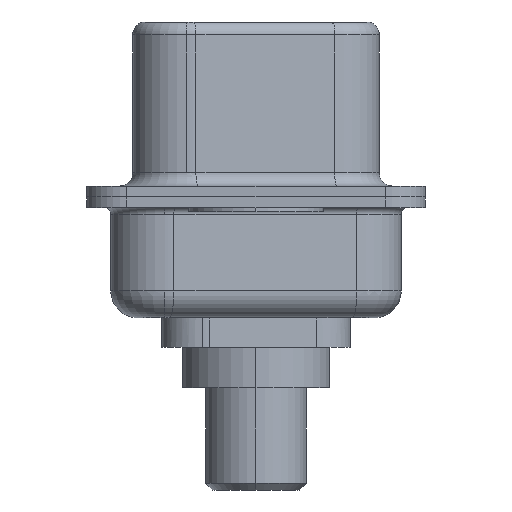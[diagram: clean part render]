
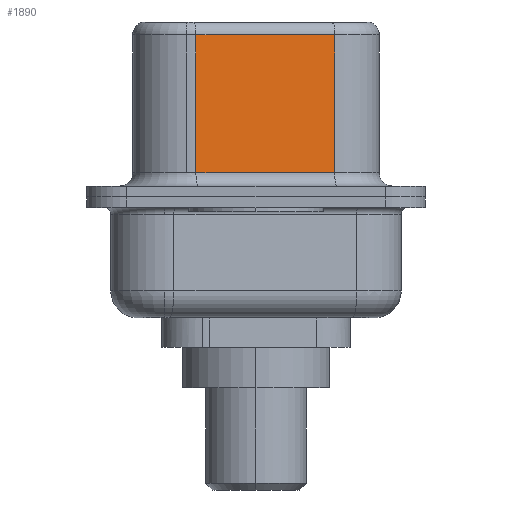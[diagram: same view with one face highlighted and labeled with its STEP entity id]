
A CAD part, left-side view. The second image highlights one B-rep face of the part: STEP entity #1890.
In plain terms, the highlighted planar face has unit normal (-0.985, -0.174, 0).
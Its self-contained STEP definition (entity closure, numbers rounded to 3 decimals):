
#310 = CARTESIAN_POINT ( 'NONE',  ( 4.585, -2.927, 6.02 ) ) ;
#383 = DIRECTION ( 'NONE',  ( -0.174, 0.985, 0. ) ) ;
#447 = DIRECTION ( 'NONE',  ( 0., 0., -1. ) ) ;
#1462 = EDGE_CURVE ( 'NONE', #12313, #4201, #1863, .T. ) ;
#1636 = ORIENTED_EDGE ( 'NONE', *, *, #1462, .T. ) ;
#1715 = VERTEX_POINT ( 'NONE', #12425 ) ;
#1863 = LINE ( 'NONE', #3931, #9402 ) ;
#1890 = ADVANCED_FACE ( 'NONE', ( #9959 ), #11284, .F. ) ;
#2063 = ORIENTED_EDGE ( 'NONE', *, *, #7433, .T. ) ;
#2094 = EDGE_LOOP ( 'NONE', ( #10419, #2063, #1636, #12164 ) ) ;
#2969 = LINE ( 'NONE', #310, #5370 ) ;
#3065 = EDGE_CURVE ( 'NONE', #4201, #1715, #9933, .T. ) ;
#3617 = EDGE_CURVE ( 'NONE', #4987, #1715, #11582, .T. ) ;
#3931 = CARTESIAN_POINT ( 'NONE',  ( 3.675, 2.233, 6.52 ) ) ;
#4201 = VERTEX_POINT ( 'NONE', #6159 ) ;
#4390 = DIRECTION ( 'NONE',  ( 0.174, -0.985, 0. ) ) ;
#4442 = CARTESIAN_POINT ( 'NONE',  ( 3.675, 2.233, 6.02 ) ) ;
#4987 = VERTEX_POINT ( 'NONE', #5252 ) ;
#5252 = CARTESIAN_POINT ( 'NONE',  ( 4.585, -2.927, 6.02 ) ) ;
#5370 = VECTOR ( 'NONE', #383, 1000. ) ;
#5829 = DIRECTION ( 'NONE',  ( -0.174, 0.985, 0. ) ) ;
#5900 = DIRECTION ( 'NONE',  ( 0.985, 0.174, 0. ) ) ;
#6159 = CARTESIAN_POINT ( 'NONE',  ( 3.675, 2.233, 0.9 ) ) ;
#6984 = CARTESIAN_POINT ( 'NONE',  ( 4.585, -2.927, 6.52 ) ) ;
#7433 = EDGE_CURVE ( 'NONE', #4987, #12313, #2969, .T. ) ;
#8253 = DIRECTION ( 'NONE',  ( 0., 0., -1. ) ) ;
#9203 = VECTOR ( 'NONE', #8253, 1000. ) ;
#9402 = VECTOR ( 'NONE', #447, 1000. ) ;
#9933 = LINE ( 'NONE', #12025, #11734 ) ;
#9959 = FACE_OUTER_BOUND ( 'NONE', #2094, .T. ) ;
#10240 = AXIS2_PLACEMENT_3D ( 'NONE', #10604, #5900, #5829 ) ;
#10419 = ORIENTED_EDGE ( 'NONE', *, *, #3617, .F. ) ;
#10604 = CARTESIAN_POINT ( 'NONE',  ( 4.585, -2.927, 6.52 ) ) ;
#11284 = PLANE ( 'NONE',  #10240 ) ;
#11582 = LINE ( 'NONE', #6984, #9203 ) ;
#11734 = VECTOR ( 'NONE', #4390, 1000. ) ;
#12025 = CARTESIAN_POINT ( 'NONE',  ( 4.585, -2.927, 0.9 ) ) ;
#12164 = ORIENTED_EDGE ( 'NONE', *, *, #3065, .T. ) ;
#12313 = VERTEX_POINT ( 'NONE', #4442 ) ;
#12425 = CARTESIAN_POINT ( 'NONE',  ( 4.585, -2.927, 0.9 ) ) ;
